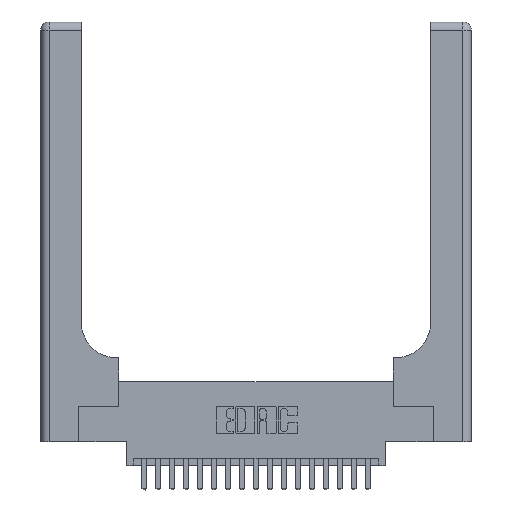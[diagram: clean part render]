
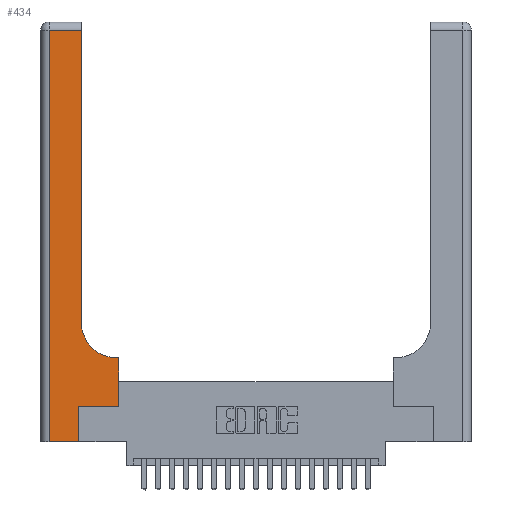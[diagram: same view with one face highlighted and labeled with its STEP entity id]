
A CAD part, top view. The second image highlights one B-rep face of the part: STEP entity #434.
In plain terms, the highlighted planar face has unit normal (0, 0, 1).
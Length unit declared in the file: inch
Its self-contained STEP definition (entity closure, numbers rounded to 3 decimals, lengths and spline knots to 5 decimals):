
#434 = ADVANCED_FACE ( 'NONE', ( #19650 ), #14772, .F. ) ;
#515 = CARTESIAN_POINT ( 'NONE',  ( 0.06, 2.94, 0.37 ) ) ;
#1033 = CARTESIAN_POINT ( 'NONE',  ( 0.2915, 0.85, 0.37 ) ) ;
#2151 = CARTESIAN_POINT ( 'NONE',  ( 0.5585, 0.25, 0.37 ) ) ;
#2191 = CARTESIAN_POINT ( 'NONE',  ( 0.06, 0., 0.37 ) ) ;
#2875 = ORIENTED_EDGE ( 'NONE', *, *, #14509, .T. ) ;
#2991 = CARTESIAN_POINT ( 'NONE',  ( 0.269, 0.25, 0.37 ) ) ;
#3762 = LINE ( 'NONE', #19472, #4314 ) ;
#3862 = ORIENTED_EDGE ( 'NONE', *, *, #12662, .T. ) ;
#4314 = VECTOR ( 'NONE', #5715, 39.37008 ) ;
#4343 = LINE ( 'NONE', #10536, #21509 ) ;
#5002 = VECTOR ( 'NONE', #19880, 39.37008 ) ;
#5444 = EDGE_CURVE ( 'NONE', #9091, #6203, #10567, .T. ) ;
#5546 = EDGE_CURVE ( 'NONE', #7859, #6811, #9585, .T. ) ;
#5715 = DIRECTION ( 'NONE',  ( 1., 0., 0. ) ) ;
#5813 = CARTESIAN_POINT ( 'NONE',  ( 0.5585, 0.25, 0.37 ) ) ;
#6203 = VERTEX_POINT ( 'NONE', #2151 ) ;
#6403 = VECTOR ( 'NONE', #14516, 39.37008 ) ;
#6554 = ORIENTED_EDGE ( 'NONE', *, *, #9835, .T. ) ;
#6714 = CARTESIAN_POINT ( 'NONE',  ( 0.2915, 0.6, 0.37 ) ) ;
#6811 = VERTEX_POINT ( 'NONE', #515 ) ;
#6855 = EDGE_CURVE ( 'NONE', #6203, #17065, #7318, .T. ) ;
#6976 = CARTESIAN_POINT ( 'NONE',  ( 0.5585, 0.6, 0.37 ) ) ;
#7318 = LINE ( 'NONE', #5813, #15871 ) ;
#7417 = CARTESIAN_POINT ( 'NONE',  ( 0.5415, 0.6, 0.37 ) ) ;
#7786 = CARTESIAN_POINT ( 'NONE',  ( 0., 2.94, 0.37 ) ) ;
#7859 = VERTEX_POINT ( 'NONE', #11609 ) ;
#8121 = ORIENTED_EDGE ( 'NONE', *, *, #6855, .T. ) ;
#8331 = DIRECTION ( 'NONE',  ( 0., 1., 0. ) ) ;
#8411 = CARTESIAN_POINT ( 'NONE',  ( 0.269, 0.25, 0.37 ) ) ;
#8914 = VERTEX_POINT ( 'NONE', #2191 ) ;
#9091 = VERTEX_POINT ( 'NONE', #2991 ) ;
#9585 = LINE ( 'NONE', #7786, #5002 ) ;
#9704 = CARTESIAN_POINT ( 'NONE',  ( 0.5415, 0.85, 0.37 ) ) ;
#9835 = EDGE_CURVE ( 'NONE', #8914, #21055, #3762, .T. ) ;
#10046 = VECTOR ( 'NONE', #17032, 39.37008 ) ;
#10132 = ORIENTED_EDGE ( 'NONE', *, *, #12945, .T. ) ;
#10536 = CARTESIAN_POINT ( 'NONE',  ( 0.06, 3., 0.37 ) ) ;
#10567 = LINE ( 'NONE', #8411, #14017 ) ;
#10944 = LINE ( 'NONE', #12711, #6403 ) ;
#11341 = CIRCLE ( 'NONE', #13886, 0.25 ) ;
#11605 = DIRECTION ( 'NONE',  ( 0., 0., -1. ) ) ;
#11609 = CARTESIAN_POINT ( 'NONE',  ( 0.2915, 2.94, 0.37 ) ) ;
#11758 = VERTEX_POINT ( 'NONE', #7417 ) ;
#12662 = EDGE_CURVE ( 'NONE', #11758, #12802, #11341, .T. ) ;
#12711 = CARTESIAN_POINT ( 'NONE',  ( 0.2915, 3., 0.37 ) ) ;
#12802 = VERTEX_POINT ( 'NONE', #1033 ) ;
#12945 = EDGE_CURVE ( 'NONE', #21055, #9091, #19986, .T. ) ;
#12968 = EDGE_LOOP ( 'NONE', ( #15789, #20472, #2875, #6554, #10132, #14274, #8121, #21821, #3862 ) ) ;
#13151 = DIRECTION ( 'NONE',  ( 1., 0., 0. ) ) ;
#13169 = VECTOR ( 'NONE', #8331, 39.37008 ) ;
#13355 = CARTESIAN_POINT ( 'NONE',  ( 0.269, 0., 0.37 ) ) ;
#13886 = AXIS2_PLACEMENT_3D ( 'NONE', #9704, #21453, #13151 ) ;
#14007 = DIRECTION ( 'NONE',  ( 0., 1., 0. ) ) ;
#14017 = VECTOR ( 'NONE', #15783, 39.37008 ) ;
#14274 = ORIENTED_EDGE ( 'NONE', *, *, #5444, .T. ) ;
#14509 = EDGE_CURVE ( 'NONE', #6811, #8914, #4343, .T. ) ;
#14516 = DIRECTION ( 'NONE',  ( 0., 1., 0. ) ) ;
#14772 = PLANE ( 'NONE',  #16300 ) ;
#15783 = DIRECTION ( 'NONE',  ( 1., 0., 0. ) ) ;
#15789 = ORIENTED_EDGE ( 'NONE', *, *, #16559, .T. ) ;
#15845 = DIRECTION ( 'NONE',  ( 0., -1., 0. ) ) ;
#15871 = VECTOR ( 'NONE', #14007, 39.37008 ) ;
#16300 = AXIS2_PLACEMENT_3D ( 'NONE', #21617, #11605, #20231 ) ;
#16559 = EDGE_CURVE ( 'NONE', #12802, #7859, #10944, .T. ) ;
#17032 = DIRECTION ( 'NONE',  ( -1., 0., 0. ) ) ;
#17065 = VERTEX_POINT ( 'NONE', #6976 ) ;
#19074 = EDGE_CURVE ( 'NONE', #17065, #11758, #20801, .T. ) ;
#19472 = CARTESIAN_POINT ( 'NONE',  ( 0., 0., 0.37 ) ) ;
#19650 = FACE_OUTER_BOUND ( 'NONE', #12968, .T. ) ;
#19880 = DIRECTION ( 'NONE',  ( -1., 0., 0. ) ) ;
#19986 = LINE ( 'NONE', #13355, #13169 ) ;
#20231 = DIRECTION ( 'NONE',  ( -1., 0., 0. ) ) ;
#20472 = ORIENTED_EDGE ( 'NONE', *, *, #5546, .T. ) ;
#20715 = CARTESIAN_POINT ( 'NONE',  ( 0.269, 0., 0.37 ) ) ;
#20801 = LINE ( 'NONE', #6714, #10046 ) ;
#21055 = VERTEX_POINT ( 'NONE', #20715 ) ;
#21453 = DIRECTION ( 'NONE',  ( 0., 0., -1. ) ) ;
#21509 = VECTOR ( 'NONE', #15845, 39.37008 ) ;
#21617 = CARTESIAN_POINT ( 'NONE',  ( 0., 3., 0.37 ) ) ;
#21821 = ORIENTED_EDGE ( 'NONE', *, *, #19074, .T. ) ;
